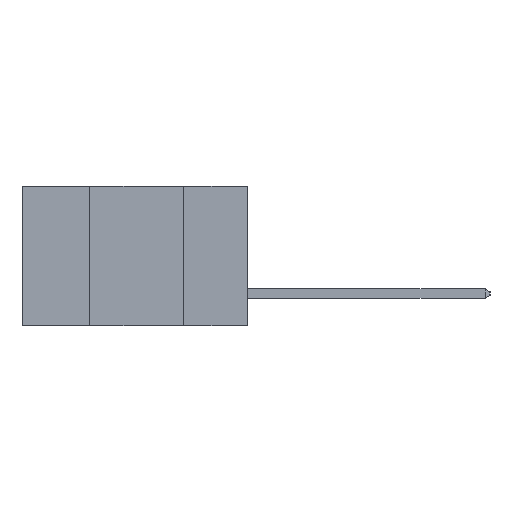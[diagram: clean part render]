
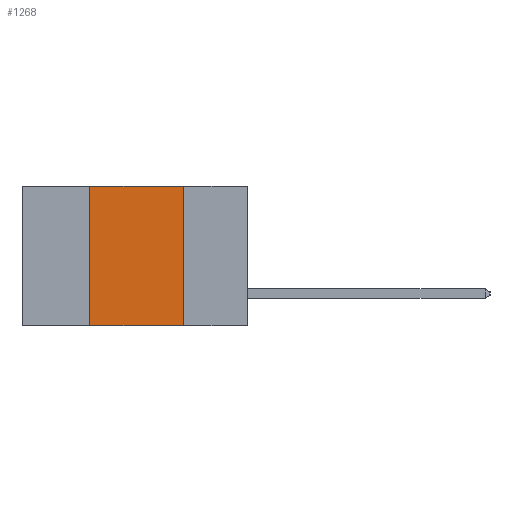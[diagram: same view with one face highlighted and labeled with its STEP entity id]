
A CAD part, left-side view. The second image highlights one B-rep face of the part: STEP entity #1268.
In plain terms, the highlighted planar face has unit normal (-1, 0, 0).
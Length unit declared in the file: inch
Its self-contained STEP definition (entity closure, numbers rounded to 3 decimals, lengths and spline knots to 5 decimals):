
#476 = VECTOR ( 'NONE', #19707, 39.37008 ) ;
#494 = CARTESIAN_POINT ( 'NONE',  ( 0., 0.6, -0.37 ) ) ;
#1268 = ADVANCED_FACE ( 'NONE', ( #8609 ), #8493, .F. ) ;
#3494 = CARTESIAN_POINT ( 'NONE',  ( 0., 0.17, -0.37 ) ) ;
#5109 = EDGE_LOOP ( 'NONE', ( #13667, #20338, #14932, #15946 ) ) ;
#5182 = LINE ( 'NONE', #6347, #8920 ) ;
#5476 = EDGE_CURVE ( 'NONE', #20030, #12056, #5738, .T. ) ;
#5738 = LINE ( 'NONE', #494, #13721 ) ;
#6096 = AXIS2_PLACEMENT_3D ( 'NONE', #18045, #9359, #16558 ) ;
#6347 = CARTESIAN_POINT ( 'NONE',  ( 0., 0.17, 0. ) ) ;
#7062 = VERTEX_POINT ( 'NONE', #11140 ) ;
#7584 = VERTEX_POINT ( 'NONE', #14120 ) ;
#8493 = PLANE ( 'NONE',  #6096 ) ;
#8609 = FACE_OUTER_BOUND ( 'NONE', #5109, .T. ) ;
#8920 = VECTOR ( 'NONE', #19043, 39.37008 ) ;
#9359 = DIRECTION ( 'NONE',  ( 1., 0., 0. ) ) ;
#10830 = EDGE_CURVE ( 'NONE', #20030, #7584, #13464, .T. ) ;
#11140 = CARTESIAN_POINT ( 'NONE',  ( 0., 0.17, 0. ) ) ;
#11423 = VECTOR ( 'NONE', #17212, 39.37008 ) ;
#11755 = EDGE_CURVE ( 'NONE', #7584, #7062, #20350, .T. ) ;
#11872 = EDGE_CURVE ( 'NONE', #7062, #12056, #5182, .T. ) ;
#12056 = VERTEX_POINT ( 'NONE', #3494 ) ;
#13464 = LINE ( 'NONE', #18126, #476 ) ;
#13515 = DIRECTION ( 'NONE',  ( 0., -1., 0. ) ) ;
#13667 = ORIENTED_EDGE ( 'NONE', *, *, #11872, .F. ) ;
#13721 = VECTOR ( 'NONE', #13515, 39.37008 ) ;
#14120 = CARTESIAN_POINT ( 'NONE',  ( 0., 0.42, 0. ) ) ;
#14932 = ORIENTED_EDGE ( 'NONE', *, *, #10830, .F. ) ;
#15557 = CARTESIAN_POINT ( 'NONE',  ( 0., 0.6, 0. ) ) ;
#15946 = ORIENTED_EDGE ( 'NONE', *, *, #5476, .T. ) ;
#16558 = DIRECTION ( 'NONE',  ( 0., 0., -1. ) ) ;
#17205 = CARTESIAN_POINT ( 'NONE',  ( 0., 0.42, -0.37 ) ) ;
#17212 = DIRECTION ( 'NONE',  ( 0., -1., 0. ) ) ;
#18045 = CARTESIAN_POINT ( 'NONE',  ( 0., 0.6, 0. ) ) ;
#18126 = CARTESIAN_POINT ( 'NONE',  ( 0., 0.42, 0. ) ) ;
#19043 = DIRECTION ( 'NONE',  ( 0., 0., -1. ) ) ;
#19707 = DIRECTION ( 'NONE',  ( 0., 0., 1. ) ) ;
#20030 = VERTEX_POINT ( 'NONE', #17205 ) ;
#20338 = ORIENTED_EDGE ( 'NONE', *, *, #11755, .F. ) ;
#20350 = LINE ( 'NONE', #15557, #11423 ) ;
